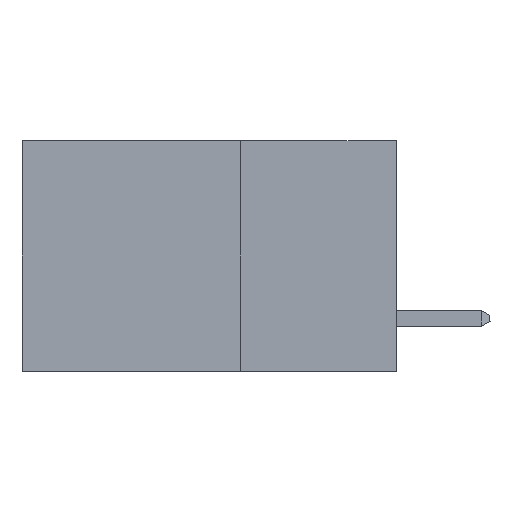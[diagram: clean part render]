
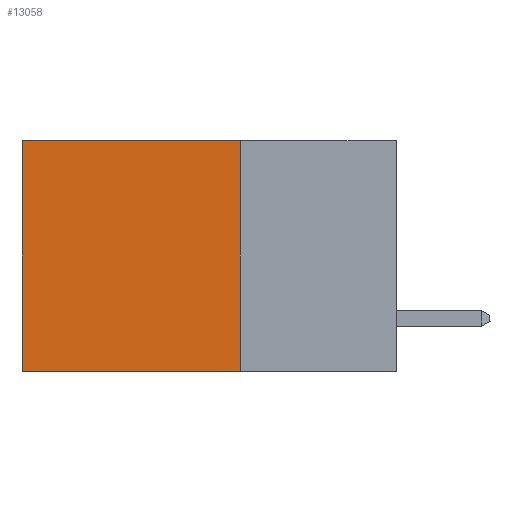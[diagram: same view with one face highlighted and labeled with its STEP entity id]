
A CAD part, left-side view. The second image highlights one B-rep face of the part: STEP entity #13058.
In plain terms, the highlighted planar face has unit normal (-1, 0, 0).
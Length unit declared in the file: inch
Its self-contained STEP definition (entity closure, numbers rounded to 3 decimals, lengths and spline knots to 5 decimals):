
#223 = VERTEX_POINT ( 'NONE', #11020 ) ;
#309 = CARTESIAN_POINT ( 'NONE',  ( 0.298, 0.25, 0. ) ) ;
#519 = CARTESIAN_POINT ( 'NONE',  ( 0.298, 0.25, 0. ) ) ;
#1370 = VECTOR ( 'NONE', #14625, 39.37008 ) ;
#1542 = DIRECTION ( 'NONE',  ( 1., 0., 0. ) ) ;
#1674 = ORIENTED_EDGE ( 'NONE', *, *, #5034, .F. ) ;
#1707 = VECTOR ( 'NONE', #4736, 39.37008 ) ;
#1971 = FACE_OUTER_BOUND ( 'NONE', #7491, .T. ) ;
#2538 = VERTEX_POINT ( 'NONE', #6768 ) ;
#2567 = EDGE_CURVE ( 'NONE', #14754, #8256, #12589, .T. ) ;
#4736 = DIRECTION ( 'NONE',  ( 0., 0., -1. ) ) ;
#5000 = VECTOR ( 'NONE', #15022, 39.37008 ) ;
#5034 = EDGE_CURVE ( 'NONE', #14754, #2538, #6485, .T. ) ;
#5671 = CARTESIAN_POINT ( 'NONE',  ( 0.298, 0.25, 0. ) ) ;
#5803 = AXIS2_PLACEMENT_3D ( 'NONE', #519, #1542, #7359 ) ;
#6485 = LINE ( 'NONE', #5671, #5000 ) ;
#6768 = CARTESIAN_POINT ( 'NONE',  ( 0.298, 0.25, -0.37 ) ) ;
#7359 = DIRECTION ( 'NONE',  ( 0., 0., -1. ) ) ;
#7491 = EDGE_LOOP ( 'NONE', ( #11917, #14105, #1674, #13564 ) ) ;
#7567 = PLANE ( 'NONE',  #5803 ) ;
#7593 = CARTESIAN_POINT ( 'NONE',  ( 0.298, 0.25, -0.37 ) ) ;
#8256 = VERTEX_POINT ( 'NONE', #12633 ) ;
#9032 = LINE ( 'NONE', #7593, #11226 ) ;
#9066 = LINE ( 'NONE', #12863, #1707 ) ;
#9718 = EDGE_CURVE ( 'NONE', #8256, #223, #9066, .T. ) ;
#9885 = CARTESIAN_POINT ( 'NONE',  ( 0.298, 0.25, 0. ) ) ;
#10109 = DIRECTION ( 'NONE',  ( 0., 1., 0. ) ) ;
#10384 = EDGE_CURVE ( 'NONE', #2538, #223, #9032, .T. ) ;
#11020 = CARTESIAN_POINT ( 'NONE',  ( 0.298, 0.6, -0.37 ) ) ;
#11226 = VECTOR ( 'NONE', #10109, 39.37008 ) ;
#11917 = ORIENTED_EDGE ( 'NONE', *, *, #9718, .T. ) ;
#12589 = LINE ( 'NONE', #9885, #1370 ) ;
#12633 = CARTESIAN_POINT ( 'NONE',  ( 0.298, 0.6, 0. ) ) ;
#12863 = CARTESIAN_POINT ( 'NONE',  ( 0.298, 0.6, 0. ) ) ;
#13058 = ADVANCED_FACE ( 'NONE', ( #1971 ), #7567, .F. ) ;
#13564 = ORIENTED_EDGE ( 'NONE', *, *, #2567, .T. ) ;
#14105 = ORIENTED_EDGE ( 'NONE', *, *, #10384, .F. ) ;
#14625 = DIRECTION ( 'NONE',  ( 0., 1., 0. ) ) ;
#14754 = VERTEX_POINT ( 'NONE', #309 ) ;
#15022 = DIRECTION ( 'NONE',  ( 0., 0., -1. ) ) ;
